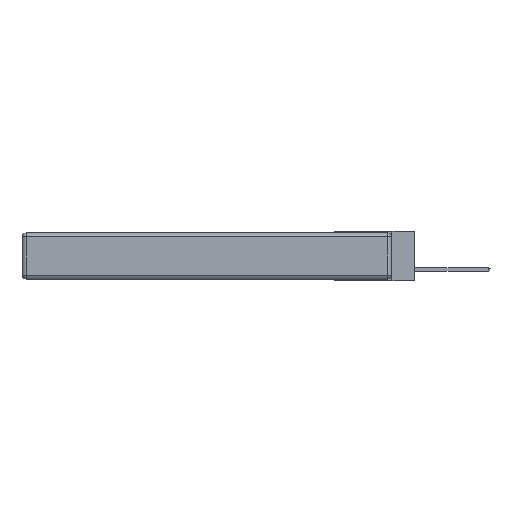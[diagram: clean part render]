
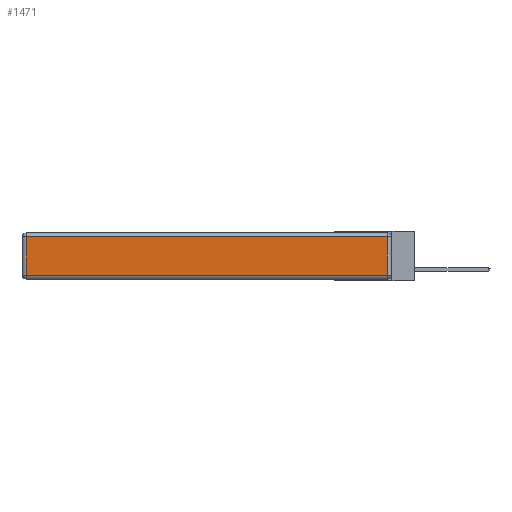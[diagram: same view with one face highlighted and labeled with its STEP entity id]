
A CAD part, left-side view. The second image highlights one B-rep face of the part: STEP entity #1471.
In plain terms, the highlighted planar face has unit normal (-1, 0, 0).
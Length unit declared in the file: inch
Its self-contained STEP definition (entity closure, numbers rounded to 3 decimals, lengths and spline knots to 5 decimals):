
#48 = VERTEX_POINT ( 'NONE', #11989 ) ;
#314 = LINE ( 'NONE', #8513, #4764 ) ;
#383 = ORIENTED_EDGE ( 'NONE', *, *, #5594, .T. ) ;
#618 = CARTESIAN_POINT ( 'NONE',  ( 0., 2.75, -0.03 ) ) ;
#682 = EDGE_CURVE ( 'NONE', #8346, #8067, #314, .T. ) ;
#742 = DIRECTION ( 'NONE',  ( 0., -1., 0. ) ) ;
#774 = VECTOR ( 'NONE', #8858, 39.37008 ) ;
#786 = CARTESIAN_POINT ( 'NONE',  ( 0., 0., -0.313 ) ) ;
#1149 = CARTESIAN_POINT ( 'NONE',  ( 0., 0.03, -0.03 ) ) ;
#1471 = ADVANCED_FACE ( 'NONE', ( #9519 ), #5759, .T. ) ;
#1662 = CARTESIAN_POINT ( 'NONE',  ( 0., 2.72, -0.313 ) ) ;
#1767 = CARTESIAN_POINT ( 'NONE',  ( 0., 0.03, -0.343 ) ) ;
#2280 = EDGE_CURVE ( 'NONE', #5754, #8346, #12094, .T. ) ;
#2763 = DIRECTION ( 'NONE',  ( -1., 0., 0. ) ) ;
#3420 = EDGE_CURVE ( 'NONE', #48, #5754, #5473, .T. ) ;
#4725 = ORIENTED_EDGE ( 'NONE', *, *, #3420, .T. ) ;
#4732 = ORIENTED_EDGE ( 'NONE', *, *, #682, .T. ) ;
#4764 = VECTOR ( 'NONE', #6667, 39.37008 ) ;
#5156 = EDGE_LOOP ( 'NONE', ( #383, #4725, #8881, #4732 ) ) ;
#5473 = LINE ( 'NONE', #1767, #11025 ) ;
#5594 = EDGE_CURVE ( 'NONE', #8067, #48, #7717, .T. ) ;
#5754 = VERTEX_POINT ( 'NONE', #1149 ) ;
#5759 = PLANE ( 'NONE',  #6410 ) ;
#6410 = AXIS2_PLACEMENT_3D ( 'NONE', #8634, #2763, #9638 ) ;
#6667 = DIRECTION ( 'NONE',  ( 0., 0., -1. ) ) ;
#7717 = LINE ( 'NONE', #786, #12132 ) ;
#8067 = VERTEX_POINT ( 'NONE', #1662 ) ;
#8346 = VERTEX_POINT ( 'NONE', #9319 ) ;
#8513 = CARTESIAN_POINT ( 'NONE',  ( 0., 2.72, -0.343 ) ) ;
#8634 = CARTESIAN_POINT ( 'NONE',  ( 0., 0., -0.343 ) ) ;
#8858 = DIRECTION ( 'NONE',  ( 0., 1., 0. ) ) ;
#8881 = ORIENTED_EDGE ( 'NONE', *, *, #2280, .T. ) ;
#9319 = CARTESIAN_POINT ( 'NONE',  ( 0., 2.72, -0.03 ) ) ;
#9519 = FACE_OUTER_BOUND ( 'NONE', #5156, .T. ) ;
#9638 = DIRECTION ( 'NONE',  ( 0., 0., 1. ) ) ;
#11025 = VECTOR ( 'NONE', #12464, 39.37008 ) ;
#11989 = CARTESIAN_POINT ( 'NONE',  ( 0., 0.03, -0.313 ) ) ;
#12094 = LINE ( 'NONE', #618, #774 ) ;
#12132 = VECTOR ( 'NONE', #742, 39.37008 ) ;
#12464 = DIRECTION ( 'NONE',  ( 0., 0., 1. ) ) ;
